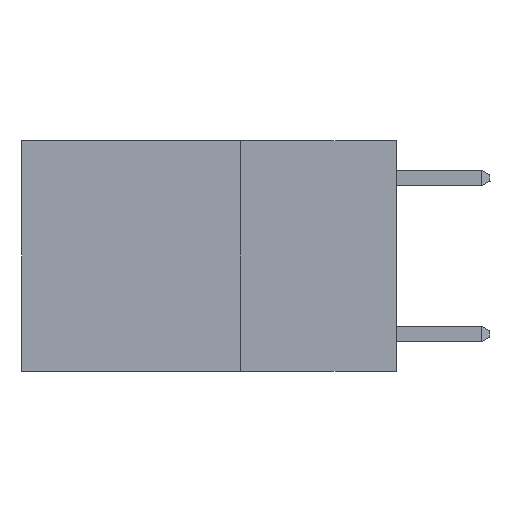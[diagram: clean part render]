
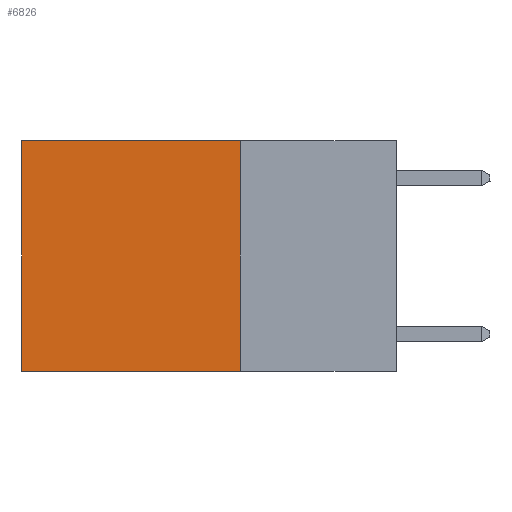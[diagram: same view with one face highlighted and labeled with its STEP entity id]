
A CAD part, left-side view. The second image highlights one B-rep face of the part: STEP entity #6826.
In plain terms, the highlighted planar face has unit normal (-1, 0, 0).
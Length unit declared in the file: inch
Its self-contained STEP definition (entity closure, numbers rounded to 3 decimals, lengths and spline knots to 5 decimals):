
#414 = EDGE_CURVE ( 'NONE', #23174, #7008, #27292, .T. ) ;
#650 = CARTESIAN_POINT ( 'NONE',  ( 0.2625, 0.25, 0. ) ) ;
#1764 = FACE_OUTER_BOUND ( 'NONE', #6538, .T. ) ;
#3721 = CARTESIAN_POINT ( 'NONE',  ( 0.2625, 0.6, 0. ) ) ;
#5359 = ORIENTED_EDGE ( 'NONE', *, *, #12681, .F. ) ;
#6538 = EDGE_LOOP ( 'NONE', ( #28087, #14387, #5359, #22946 ) ) ;
#6826 = ADVANCED_FACE ( 'NONE', ( #1764 ), #7333, .F. ) ;
#7008 = VERTEX_POINT ( 'NONE', #16699 ) ;
#7333 = PLANE ( 'NONE',  #10032 ) ;
#8410 = DIRECTION ( 'NONE',  ( 0., 0., -1. ) ) ;
#8965 = CARTESIAN_POINT ( 'NONE',  ( 0.2625, 0.6, 0. ) ) ;
#10032 = AXIS2_PLACEMENT_3D ( 'NONE', #19665, #14834, #22070 ) ;
#12681 = EDGE_CURVE ( 'NONE', #26615, #21029, #19757, .T. ) ;
#14370 = VECTOR ( 'NONE', #8410, 39.37008 ) ;
#14387 = ORIENTED_EDGE ( 'NONE', *, *, #17877, .F. ) ;
#14834 = DIRECTION ( 'NONE',  ( 1., 0., 0. ) ) ;
#16699 = CARTESIAN_POINT ( 'NONE',  ( 0.2625, 0.6, -0.37 ) ) ;
#17772 = VECTOR ( 'NONE', #23465, 39.37008 ) ;
#17877 = EDGE_CURVE ( 'NONE', #21029, #7008, #25622, .T. ) ;
#19454 = CARTESIAN_POINT ( 'NONE',  ( 0.2625, 0.25, -0.37 ) ) ;
#19665 = CARTESIAN_POINT ( 'NONE',  ( 0.2625, 0.25, 0. ) ) ;
#19757 = LINE ( 'NONE', #650, #14370 ) ;
#20715 = DIRECTION ( 'NONE',  ( 0., 1., 0. ) ) ;
#21029 = VERTEX_POINT ( 'NONE', #21693 ) ;
#21397 = EDGE_CURVE ( 'NONE', #26615, #23174, #30317, .T. ) ;
#21693 = CARTESIAN_POINT ( 'NONE',  ( 0.2625, 0.25, -0.37 ) ) ;
#22070 = DIRECTION ( 'NONE',  ( 0., 0., -1. ) ) ;
#22729 = CARTESIAN_POINT ( 'NONE',  ( 0.2625, 0.25, 0. ) ) ;
#22946 = ORIENTED_EDGE ( 'NONE', *, *, #21397, .T. ) ;
#23174 = VERTEX_POINT ( 'NONE', #8965 ) ;
#23465 = DIRECTION ( 'NONE',  ( 0., 0., -1. ) ) ;
#24023 = DIRECTION ( 'NONE',  ( 0., 1., 0. ) ) ;
#24918 = VECTOR ( 'NONE', #20715, 39.37008 ) ;
#25622 = LINE ( 'NONE', #19454, #28309 ) ;
#26615 = VERTEX_POINT ( 'NONE', #27247 ) ;
#27247 = CARTESIAN_POINT ( 'NONE',  ( 0.2625, 0.25, 0. ) ) ;
#27292 = LINE ( 'NONE', #3721, #17772 ) ;
#28087 = ORIENTED_EDGE ( 'NONE', *, *, #414, .T. ) ;
#28309 = VECTOR ( 'NONE', #24023, 39.37008 ) ;
#30317 = LINE ( 'NONE', #22729, #24918 ) ;
